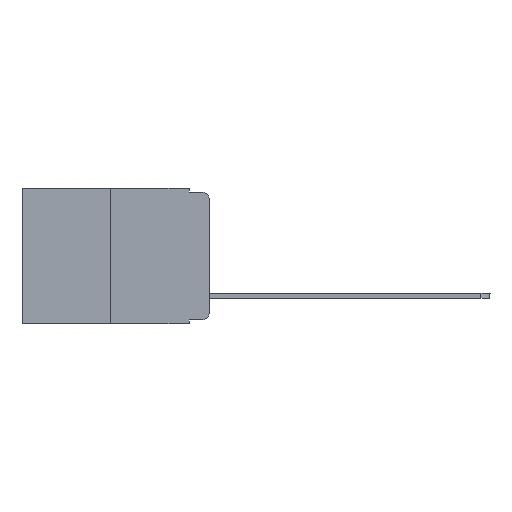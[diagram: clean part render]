
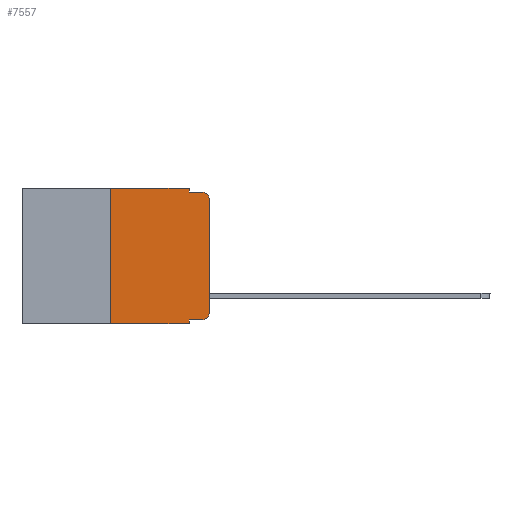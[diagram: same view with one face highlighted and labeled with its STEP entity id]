
A CAD part, left-side view. The second image highlights one B-rep face of the part: STEP entity #7557.
In plain terms, the highlighted planar face has unit normal (-1, 0, 0).
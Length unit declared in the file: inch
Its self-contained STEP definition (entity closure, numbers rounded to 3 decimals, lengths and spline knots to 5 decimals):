
#89 = CARTESIAN_POINT ( 'NONE',  ( 0., 0., -0.03 ) ) ;
#203 = AXIS2_PLACEMENT_3D ( 'NONE', #8913, #9774, #4776 ) ;
#350 = VECTOR ( 'NONE', #1220, 39.37008 ) ;
#562 = AXIS2_PLACEMENT_3D ( 'NONE', #12055, #8093, #11959 ) ;
#787 = ORIENTED_EDGE ( 'NONE', *, *, #4126, .F. ) ;
#854 = PLANE ( 'NONE',  #11010 ) ;
#942 = EDGE_CURVE ( 'NONE', #3152, #1296, #7057, .T. ) ;
#1193 = EDGE_CURVE ( 'NONE', #1347, #6391, #4318, .T. ) ;
#1220 = DIRECTION ( 'NONE',  ( 0., 0., -1. ) ) ;
#1296 = VERTEX_POINT ( 'NONE', #7488 ) ;
#1347 = VERTEX_POINT ( 'NONE', #11675 ) ;
#1577 = VECTOR ( 'NONE', #4899, 39.37008 ) ;
#1605 = CIRCLE ( 'NONE', #203, 0.02 ) ;
#2106 = VERTEX_POINT ( 'NONE', #7232 ) ;
#2603 = VERTEX_POINT ( 'NONE', #4619 ) ;
#2633 = ORIENTED_EDGE ( 'NONE', *, *, #942, .F. ) ;
#2759 = EDGE_CURVE ( 'NONE', #1347, #12540, #11044, .T. ) ;
#2875 = CARTESIAN_POINT ( 'NONE',  ( 0., 0.473, -0.343 ) ) ;
#3152 = VERTEX_POINT ( 'NONE', #4877 ) ;
#3493 = EDGE_CURVE ( 'NONE', #12540, #3813, #1605, .T. ) ;
#3677 = VECTOR ( 'NONE', #3886, 39.37008 ) ;
#3813 = VERTEX_POINT ( 'NONE', #6565 ) ;
#3886 = DIRECTION ( 'NONE',  ( 0., -1., 0. ) ) ;
#3914 = ORIENTED_EDGE ( 'NONE', *, *, #6728, .T. ) ;
#4115 = CIRCLE ( 'NONE', #562, 0.02 ) ;
#4126 = EDGE_CURVE ( 'NONE', #2106, #3152, #4164, .T. ) ;
#4164 = LINE ( 'NONE', #8843, #1577 ) ;
#4318 = LINE ( 'NONE', #11129, #10676 ) ;
#4470 = EDGE_LOOP ( 'NONE', ( #8694, #3914, #6866, #9081, #2633, #787, #10168, #11925, #5694, #8639 ) ) ;
#4619 = CARTESIAN_POINT ( 'NONE',  ( 0., 0.02, -0.01 ) ) ;
#4776 = DIRECTION ( 'NONE',  ( 0., 0., -1. ) ) ;
#4798 = CARTESIAN_POINT ( 'NONE',  ( 0., 0.02, -0.333 ) ) ;
#4877 = CARTESIAN_POINT ( 'NONE',  ( 0., 0.25, 0. ) ) ;
#4899 = DIRECTION ( 'NONE',  ( 0., 0., 1. ) ) ;
#5149 = DIRECTION ( 'NONE',  ( 0., -1., 0. ) ) ;
#5384 = VECTOR ( 'NONE', #11075, 39.37008 ) ;
#5622 = EDGE_CURVE ( 'NONE', #12731, #2603, #6856, .T. ) ;
#5694 = ORIENTED_EDGE ( 'NONE', *, *, #2759, .T. ) ;
#6186 = CARTESIAN_POINT ( 'NONE',  ( 0., 0.051, 0. ) ) ;
#6207 = LINE ( 'NONE', #2875, #5384 ) ;
#6391 = VERTEX_POINT ( 'NONE', #9418 ) ;
#6407 = CARTESIAN_POINT ( 'NONE',  ( 0., 0.051, -0.01 ) ) ;
#6565 = CARTESIAN_POINT ( 'NONE',  ( 0., 0., -0.313 ) ) ;
#6728 = EDGE_CURVE ( 'NONE', #10181, #2603, #4115, .T. ) ;
#6744 = EDGE_CURVE ( 'NONE', #2106, #6391, #6207, .T. ) ;
#6824 = EDGE_CURVE ( 'NONE', #3813, #10181, #8115, .T. ) ;
#6856 = LINE ( 'NONE', #10109, #7828 ) ;
#6866 = ORIENTED_EDGE ( 'NONE', *, *, #5622, .F. ) ;
#7034 = CARTESIAN_POINT ( 'NONE',  ( 0., 0.051, -0.333 ) ) ;
#7057 = LINE ( 'NONE', #9033, #3677 ) ;
#7149 = DIRECTION ( 'NONE',  ( 0., 0., -1. ) ) ;
#7232 = CARTESIAN_POINT ( 'NONE',  ( 0., 0.25, -0.343 ) ) ;
#7488 = CARTESIAN_POINT ( 'NONE',  ( 0., 0.051, 0. ) ) ;
#7557 = ADVANCED_FACE ( 'NONE', ( #9363 ), #854, .F. ) ;
#7828 = VECTOR ( 'NONE', #12081, 39.37008 ) ;
#7961 = CARTESIAN_POINT ( 'NONE',  ( 0., 0.473, 0. ) ) ;
#8093 = DIRECTION ( 'NONE',  ( -1., 0., 0. ) ) ;
#8115 = LINE ( 'NONE', #10162, #12535 ) ;
#8345 = DIRECTION ( 'NONE',  ( 1., 0., 0. ) ) ;
#8639 = ORIENTED_EDGE ( 'NONE', *, *, #3493, .T. ) ;
#8694 = ORIENTED_EDGE ( 'NONE', *, *, #6824, .T. ) ;
#8843 = CARTESIAN_POINT ( 'NONE',  ( 0., 0.25, 0. ) ) ;
#8913 = CARTESIAN_POINT ( 'NONE',  ( 0., 0.02, -0.313 ) ) ;
#9033 = CARTESIAN_POINT ( 'NONE',  ( 0., 0.473, 0. ) ) ;
#9081 = ORIENTED_EDGE ( 'NONE', *, *, #11527, .F. ) ;
#9162 = VECTOR ( 'NONE', #5149, 39.37008 ) ;
#9363 = FACE_OUTER_BOUND ( 'NONE', #4470, .T. ) ;
#9418 = CARTESIAN_POINT ( 'NONE',  ( 0., 0.051, -0.343 ) ) ;
#9774 = DIRECTION ( 'NONE',  ( -1., 0., 0. ) ) ;
#10109 = CARTESIAN_POINT ( 'NONE',  ( 0., 0.051, -0.01 ) ) ;
#10128 = LINE ( 'NONE', #6186, #350 ) ;
#10162 = CARTESIAN_POINT ( 'NONE',  ( 0., 0., 0. ) ) ;
#10168 = ORIENTED_EDGE ( 'NONE', *, *, #6744, .T. ) ;
#10181 = VERTEX_POINT ( 'NONE', #89 ) ;
#10676 = VECTOR ( 'NONE', #7149, 39.37008 ) ;
#11010 = AXIS2_PLACEMENT_3D ( 'NONE', #7961, #8345, #12585 ) ;
#11044 = LINE ( 'NONE', #7034, #9162 ) ;
#11075 = DIRECTION ( 'NONE',  ( 0., -1., 0. ) ) ;
#11129 = CARTESIAN_POINT ( 'NONE',  ( 0., 0.051, 0. ) ) ;
#11206 = DIRECTION ( 'NONE',  ( 0., 0., 1. ) ) ;
#11527 = EDGE_CURVE ( 'NONE', #1296, #12731, #10128, .T. ) ;
#11675 = CARTESIAN_POINT ( 'NONE',  ( 0., 0.051, -0.333 ) ) ;
#11925 = ORIENTED_EDGE ( 'NONE', *, *, #1193, .F. ) ;
#11959 = DIRECTION ( 'NONE',  ( 0., 0., -1. ) ) ;
#12055 = CARTESIAN_POINT ( 'NONE',  ( 0., 0.02, -0.03 ) ) ;
#12081 = DIRECTION ( 'NONE',  ( 0., -1., 0. ) ) ;
#12535 = VECTOR ( 'NONE', #11206, 39.37008 ) ;
#12540 = VERTEX_POINT ( 'NONE', #4798 ) ;
#12585 = DIRECTION ( 'NONE',  ( 0., 0., -1. ) ) ;
#12731 = VERTEX_POINT ( 'NONE', #6407 ) ;
